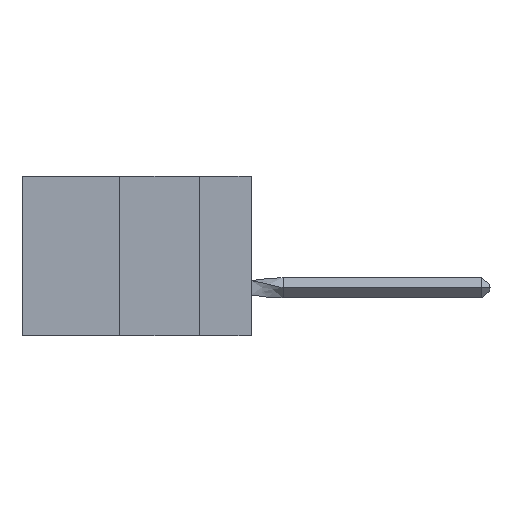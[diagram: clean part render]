
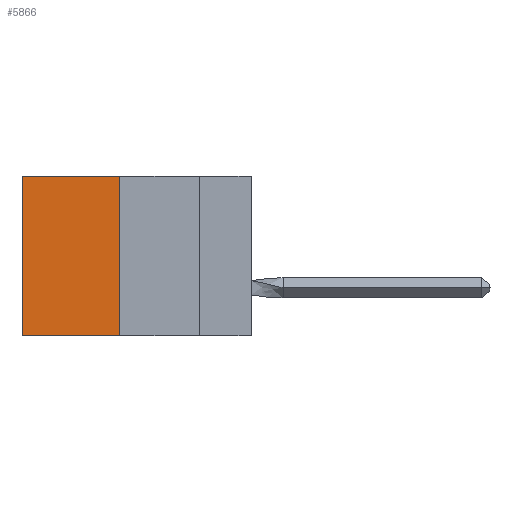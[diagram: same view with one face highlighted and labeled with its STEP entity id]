
A CAD part, left-side view. The second image highlights one B-rep face of the part: STEP entity #5866.
In plain terms, the highlighted planar face has unit normal (-1, 0, 0).
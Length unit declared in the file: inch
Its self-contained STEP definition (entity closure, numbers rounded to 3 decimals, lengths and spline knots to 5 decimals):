
#13 = EDGE_LOOP ( 'NONE', ( #13838, #17794, #13171, #3489 ) ) ;
#322 = LINE ( 'NONE', #14916, #13107 ) ;
#368 = LINE ( 'NONE', #2424, #2035 ) ;
#1022 = CARTESIAN_POINT ( 'NONE',  ( 0.305, 0.413, 0. ) ) ;
#1786 = PLANE ( 'NONE',  #14310 ) ;
#1856 = DIRECTION ( 'NONE',  ( 0., 0., -1. ) ) ;
#2035 = VECTOR ( 'NONE', #21830, 39.37008 ) ;
#2240 = FACE_OUTER_BOUND ( 'NONE', #13, .T. ) ;
#2424 = CARTESIAN_POINT ( 'NONE',  ( 0.305, 0.72, -0.5 ) ) ;
#3489 = ORIENTED_EDGE ( 'NONE', *, *, #12379, .T. ) ;
#5579 = EDGE_CURVE ( 'NONE', #5756, #20354, #322, .T. ) ;
#5756 = VERTEX_POINT ( 'NONE', #22064 ) ;
#5866 = ADVANCED_FACE ( 'NONE', ( #2240 ), #1786, .F. ) ;
#7806 = LINE ( 'NONE', #14346, #15176 ) ;
#8926 = EDGE_CURVE ( 'NONE', #20354, #14343, #7806, .T. ) ;
#9509 = LINE ( 'NONE', #1022, #12473 ) ;
#10507 = DIRECTION ( 'NONE',  ( 1., 0., 0. ) ) ;
#10651 = CARTESIAN_POINT ( 'NONE',  ( 0.305, 0.413, -0.5 ) ) ;
#10821 = DIRECTION ( 'NONE',  ( 0., 1., 0. ) ) ;
#11964 = VERTEX_POINT ( 'NONE', #19447 ) ;
#12379 = EDGE_CURVE ( 'NONE', #5756, #11964, #9509, .T. ) ;
#12473 = VECTOR ( 'NONE', #13196, 39.37008 ) ;
#13107 = VECTOR ( 'NONE', #16856, 39.37008 ) ;
#13171 = ORIENTED_EDGE ( 'NONE', *, *, #5579, .F. ) ;
#13196 = DIRECTION ( 'NONE',  ( 0., 1., 0. ) ) ;
#13700 = CARTESIAN_POINT ( 'NONE',  ( 0.305, 0.413, -0.5 ) ) ;
#13838 = ORIENTED_EDGE ( 'NONE', *, *, #21227, .T. ) ;
#14310 = AXIS2_PLACEMENT_3D ( 'NONE', #10651, #10507, #1856 ) ;
#14343 = VERTEX_POINT ( 'NONE', #18756 ) ;
#14346 = CARTESIAN_POINT ( 'NONE',  ( 0.305, 0.413, -0.5 ) ) ;
#14916 = CARTESIAN_POINT ( 'NONE',  ( 0.305, 0.413, -0.5 ) ) ;
#15176 = VECTOR ( 'NONE', #10821, 39.37008 ) ;
#16856 = DIRECTION ( 'NONE',  ( 0., 0., -1. ) ) ;
#17794 = ORIENTED_EDGE ( 'NONE', *, *, #8926, .F. ) ;
#18756 = CARTESIAN_POINT ( 'NONE',  ( 0.305, 0.72, -0.5 ) ) ;
#19447 = CARTESIAN_POINT ( 'NONE',  ( 0.305, 0.72, 0. ) ) ;
#20354 = VERTEX_POINT ( 'NONE', #13700 ) ;
#21227 = EDGE_CURVE ( 'NONE', #11964, #14343, #368, .T. ) ;
#21830 = DIRECTION ( 'NONE',  ( 0., 0., -1. ) ) ;
#22064 = CARTESIAN_POINT ( 'NONE',  ( 0.305, 0.413, 0. ) ) ;
